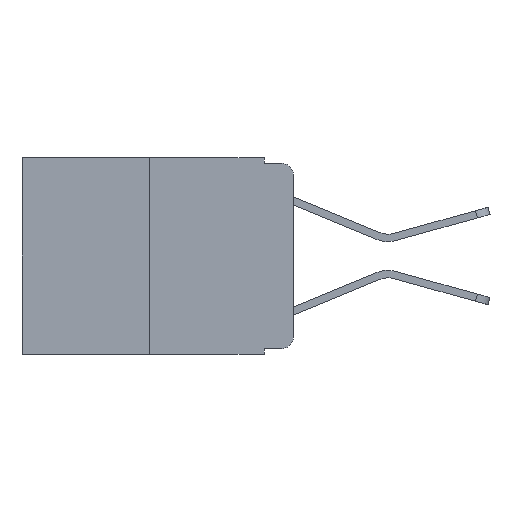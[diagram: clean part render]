
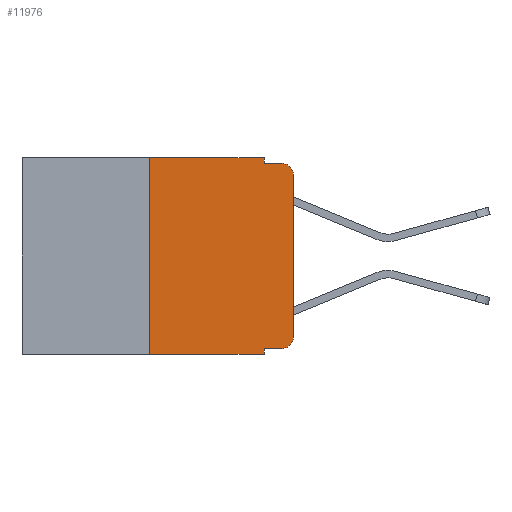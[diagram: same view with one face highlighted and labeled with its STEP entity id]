
A CAD part, left-side view. The second image highlights one B-rep face of the part: STEP entity #11976.
In plain terms, the highlighted planar face has unit normal (-1, 0, 0).
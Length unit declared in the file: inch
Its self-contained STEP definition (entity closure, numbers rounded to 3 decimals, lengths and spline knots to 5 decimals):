
#561 = CARTESIAN_POINT ( 'NONE',  ( 0., 0.25, 0. ) ) ;
#677 = CARTESIAN_POINT ( 'NONE',  ( 0., 0., -0.03 ) ) ;
#774 = ORIENTED_EDGE ( 'NONE', *, *, #3132, .T. ) ;
#805 = ORIENTED_EDGE ( 'NONE', *, *, #5323, .T. ) ;
#823 = CARTESIAN_POINT ( 'NONE',  ( 0., 0.02, -0.333 ) ) ;
#910 = CARTESIAN_POINT ( 'NONE',  ( 0., 0.25, -0.343 ) ) ;
#1227 = ORIENTED_EDGE ( 'NONE', *, *, #11920, .F. ) ;
#1579 = LINE ( 'NONE', #4319, #12332 ) ;
#2009 = CARTESIAN_POINT ( 'NONE',  ( 0., 0.051, 0. ) ) ;
#2194 = VECTOR ( 'NONE', #5063, 39.37008 ) ;
#2236 = ORIENTED_EDGE ( 'NONE', *, *, #5409, .T. ) ;
#2264 = DIRECTION ( 'NONE',  ( -1., 0., 0. ) ) ;
#2677 = CARTESIAN_POINT ( 'NONE',  ( 0., 0., -0.313 ) ) ;
#2937 = VERTEX_POINT ( 'NONE', #11424 ) ;
#3132 = EDGE_CURVE ( 'NONE', #2937, #7852, #10711, .T. ) ;
#3379 = AXIS2_PLACEMENT_3D ( 'NONE', #8004, #2264, #11769 ) ;
#3764 = EDGE_CURVE ( 'NONE', #9030, #5916, #1579, .T. ) ;
#3820 = VECTOR ( 'NONE', #9308, 39.37008 ) ;
#3833 = DIRECTION ( 'NONE',  ( -1., 0., 0. ) ) ;
#3903 = CARTESIAN_POINT ( 'NONE',  ( 0., 0.051, -0.333 ) ) ;
#3980 = VECTOR ( 'NONE', #7105, 39.37008 ) ;
#4103 = ORIENTED_EDGE ( 'NONE', *, *, #3764, .F. ) ;
#4110 = CARTESIAN_POINT ( 'NONE',  ( 0., 0.051, -0.01 ) ) ;
#4186 = AXIS2_PLACEMENT_3D ( 'NONE', #6761, #3833, #9816 ) ;
#4319 = CARTESIAN_POINT ( 'NONE',  ( 0., 0.473, 0. ) ) ;
#4388 = VECTOR ( 'NONE', #8687, 39.37008 ) ;
#4436 = VECTOR ( 'NONE', #5458, 39.37008 ) ;
#4611 = EDGE_CURVE ( 'NONE', #2937, #6208, #10731, .T. ) ;
#4621 = DIRECTION ( 'NONE',  ( 0., 0., -1. ) ) ;
#4674 = ORIENTED_EDGE ( 'NONE', *, *, #7177, .F. ) ;
#4808 = FACE_OUTER_BOUND ( 'NONE', #10691, .T. ) ;
#4842 = EDGE_CURVE ( 'NONE', #7852, #8329, #7040, .T. ) ;
#5063 = DIRECTION ( 'NONE',  ( 0., -1., 0. ) ) ;
#5244 = ORIENTED_EDGE ( 'NONE', *, *, #4842, .T. ) ;
#5323 = EDGE_CURVE ( 'NONE', #8329, #9629, #11702, .T. ) ;
#5387 = LINE ( 'NONE', #10297, #4436 ) ;
#5409 = EDGE_CURVE ( 'NONE', #9629, #7127, #7655, .T. ) ;
#5458 = DIRECTION ( 'NONE',  ( 0., 0., 1. ) ) ;
#5563 = LINE ( 'NONE', #9472, #9876 ) ;
#5842 = CARTESIAN_POINT ( 'NONE',  ( 0., 0., 0. ) ) ;
#5916 = VERTEX_POINT ( 'NONE', #6985 ) ;
#6208 = VERTEX_POINT ( 'NONE', #11672 ) ;
#6235 = CARTESIAN_POINT ( 'NONE',  ( 0., 0.473, -0.343 ) ) ;
#6761 = CARTESIAN_POINT ( 'NONE',  ( 0., 0.02, -0.313 ) ) ;
#6849 = DIRECTION ( 'NONE',  ( 0., 0., -1. ) ) ;
#6853 = ORIENTED_EDGE ( 'NONE', *, *, #4611, .F. ) ;
#6931 = EDGE_CURVE ( 'NONE', #11950, #9030, #5387, .T. ) ;
#6985 = CARTESIAN_POINT ( 'NONE',  ( 0., 0.051, 0. ) ) ;
#7040 = CIRCLE ( 'NONE', #4186, 0.02 ) ;
#7105 = DIRECTION ( 'NONE',  ( 0., 0., -1. ) ) ;
#7127 = VERTEX_POINT ( 'NONE', #11936 ) ;
#7177 = EDGE_CURVE ( 'NONE', #8422, #7127, #9977, .T. ) ;
#7244 = VECTOR ( 'NONE', #12528, 39.37008 ) ;
#7655 = CIRCLE ( 'NONE', #3379, 0.02 ) ;
#7852 = VERTEX_POINT ( 'NONE', #823 ) ;
#8004 = CARTESIAN_POINT ( 'NONE',  ( 0., 0.02, -0.03 ) ) ;
#8160 = AXIS2_PLACEMENT_3D ( 'NONE', #11678, #9727, #6849 ) ;
#8329 = VERTEX_POINT ( 'NONE', #2677 ) ;
#8349 = ORIENTED_EDGE ( 'NONE', *, *, #6931, .F. ) ;
#8422 = VERTEX_POINT ( 'NONE', #10491 ) ;
#8633 = PLANE ( 'NONE',  #8160 ) ;
#8687 = DIRECTION ( 'NONE',  ( 0., -1., 0. ) ) ;
#9030 = VERTEX_POINT ( 'NONE', #561 ) ;
#9308 = DIRECTION ( 'NONE',  ( 0., -1., 0. ) ) ;
#9472 = CARTESIAN_POINT ( 'NONE',  ( 0., 0.051, 0. ) ) ;
#9526 = EDGE_CURVE ( 'NONE', #11950, #6208, #10189, .T. ) ;
#9629 = VERTEX_POINT ( 'NONE', #677 ) ;
#9654 = ORIENTED_EDGE ( 'NONE', *, *, #9526, .T. ) ;
#9727 = DIRECTION ( 'NONE',  ( 1., 0., 0. ) ) ;
#9816 = DIRECTION ( 'NONE',  ( 0., 0., -1. ) ) ;
#9876 = VECTOR ( 'NONE', #4621, 39.37008 ) ;
#9977 = LINE ( 'NONE', #4110, #2194 ) ;
#10189 = LINE ( 'NONE', #6235, #3820 ) ;
#10297 = CARTESIAN_POINT ( 'NONE',  ( 0., 0.25, 0. ) ) ;
#10491 = CARTESIAN_POINT ( 'NONE',  ( 0., 0.051, -0.01 ) ) ;
#10691 = EDGE_LOOP ( 'NONE', ( #805, #2236, #4674, #1227, #4103, #8349, #9654, #6853, #774, #5244 ) ) ;
#10711 = LINE ( 'NONE', #3903, #4388 ) ;
#10731 = LINE ( 'NONE', #2009, #3980 ) ;
#11125 = DIRECTION ( 'NONE',  ( 0., -1., 0. ) ) ;
#11424 = CARTESIAN_POINT ( 'NONE',  ( 0., 0.051, -0.333 ) ) ;
#11672 = CARTESIAN_POINT ( 'NONE',  ( 0., 0.051, -0.343 ) ) ;
#11678 = CARTESIAN_POINT ( 'NONE',  ( 0., 0.473, 0. ) ) ;
#11702 = LINE ( 'NONE', #5842, #7244 ) ;
#11769 = DIRECTION ( 'NONE',  ( 0., 0., -1. ) ) ;
#11920 = EDGE_CURVE ( 'NONE', #5916, #8422, #5563, .T. ) ;
#11936 = CARTESIAN_POINT ( 'NONE',  ( 0., 0.02, -0.01 ) ) ;
#11950 = VERTEX_POINT ( 'NONE', #910 ) ;
#11976 = ADVANCED_FACE ( 'NONE', ( #4808 ), #8633, .F. ) ;
#12332 = VECTOR ( 'NONE', #11125, 39.37008 ) ;
#12528 = DIRECTION ( 'NONE',  ( 0., 0., 1. ) ) ;
